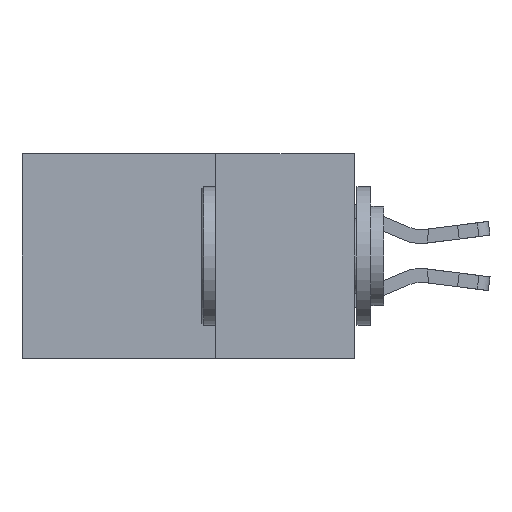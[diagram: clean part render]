
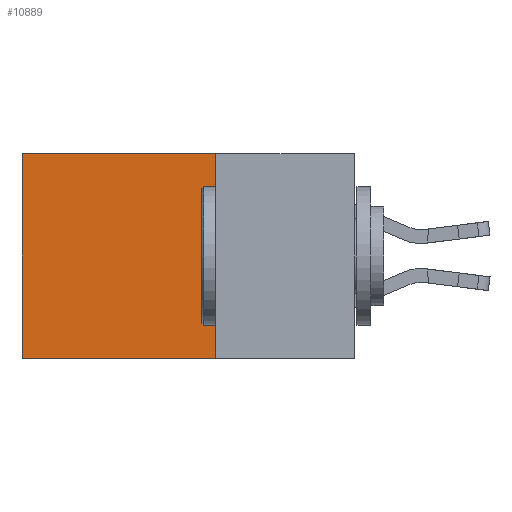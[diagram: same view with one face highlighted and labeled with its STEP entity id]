
A CAD part, left-side view. The second image highlights one B-rep face of the part: STEP entity #10889.
In plain terms, the highlighted planar face has unit normal (-1, 0, 0).
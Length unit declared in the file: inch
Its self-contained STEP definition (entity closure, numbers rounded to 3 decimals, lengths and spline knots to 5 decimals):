
#1763 = EDGE_LOOP ( 'NONE', ( #16170, #22330, #15768, #17515 ) ) ;
#1869 = PLANE ( 'NONE',  #23107 ) ;
#3036 = DIRECTION ( 'NONE',  ( 0., 1., 0. ) ) ;
#3303 = CARTESIAN_POINT ( 'NONE',  ( 0.298, 0.25, -0.37 ) ) ;
#4510 = VERTEX_POINT ( 'NONE', #14389 ) ;
#4543 = LINE ( 'NONE', #3303, #10527 ) ;
#5570 = DIRECTION ( 'NONE',  ( 0., 0., -1. ) ) ;
#6278 = EDGE_CURVE ( 'NONE', #7313, #4510, #23803, .T. ) ;
#6696 = LINE ( 'NONE', #8971, #14192 ) ;
#7094 = VECTOR ( 'NONE', #10741, 39.37008 ) ;
#7313 = VERTEX_POINT ( 'NONE', #13944 ) ;
#7342 = CARTESIAN_POINT ( 'NONE',  ( 0.298, 0.6, 0. ) ) ;
#7516 = DIRECTION ( 'NONE',  ( 0., 0., -1. ) ) ;
#8971 = CARTESIAN_POINT ( 'NONE',  ( 0.298, 0.25, 0. ) ) ;
#9771 = CARTESIAN_POINT ( 'NONE',  ( 0.298, 0.25, 0. ) ) ;
#10527 = VECTOR ( 'NONE', #3036, 39.37008 ) ;
#10741 = DIRECTION ( 'NONE',  ( 0., 0., -1. ) ) ;
#10889 = ADVANCED_FACE ( 'NONE', ( #15817 ), #1869, .F. ) ;
#12388 = VERTEX_POINT ( 'NONE', #25188 ) ;
#12643 = CARTESIAN_POINT ( 'NONE',  ( 0.298, 0.25, 0. ) ) ;
#12873 = EDGE_CURVE ( 'NONE', #25246, #7313, #6696, .T. ) ;
#13944 = CARTESIAN_POINT ( 'NONE',  ( 0.298, 0.6, 0. ) ) ;
#14192 = VECTOR ( 'NONE', #22859, 39.37008 ) ;
#14389 = CARTESIAN_POINT ( 'NONE',  ( 0.298, 0.6, -0.37 ) ) ;
#14565 = LINE ( 'NONE', #12643, #7094 ) ;
#15768 = ORIENTED_EDGE ( 'NONE', *, *, #17745, .F. ) ;
#15817 = FACE_OUTER_BOUND ( 'NONE', #1763, .T. ) ;
#16170 = ORIENTED_EDGE ( 'NONE', *, *, #6278, .T. ) ;
#17515 = ORIENTED_EDGE ( 'NONE', *, *, #12873, .T. ) ;
#17745 = EDGE_CURVE ( 'NONE', #25246, #12388, #14565, .T. ) ;
#19448 = CARTESIAN_POINT ( 'NONE',  ( 0.298, 0.25, 0. ) ) ;
#19795 = VECTOR ( 'NONE', #5570, 39.37008 ) ;
#22330 = ORIENTED_EDGE ( 'NONE', *, *, #23336, .F. ) ;
#22859 = DIRECTION ( 'NONE',  ( 0., 1., 0. ) ) ;
#23107 = AXIS2_PLACEMENT_3D ( 'NONE', #19448, #23669, #7516 ) ;
#23336 = EDGE_CURVE ( 'NONE', #12388, #4510, #4543, .T. ) ;
#23669 = DIRECTION ( 'NONE',  ( 1., 0., 0. ) ) ;
#23803 = LINE ( 'NONE', #7342, #19795 ) ;
#25188 = CARTESIAN_POINT ( 'NONE',  ( 0.298, 0.25, -0.37 ) ) ;
#25246 = VERTEX_POINT ( 'NONE', #9771 ) ;
